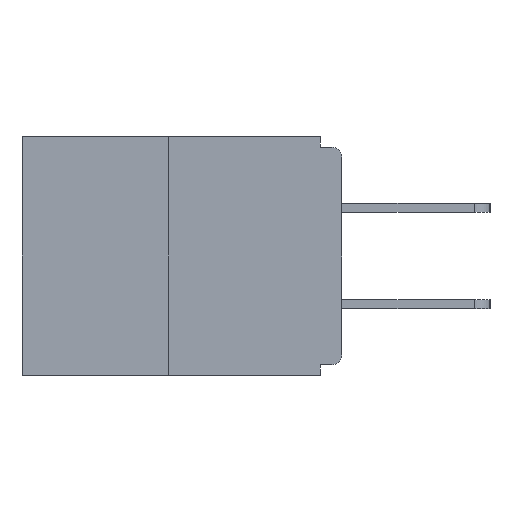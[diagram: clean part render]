
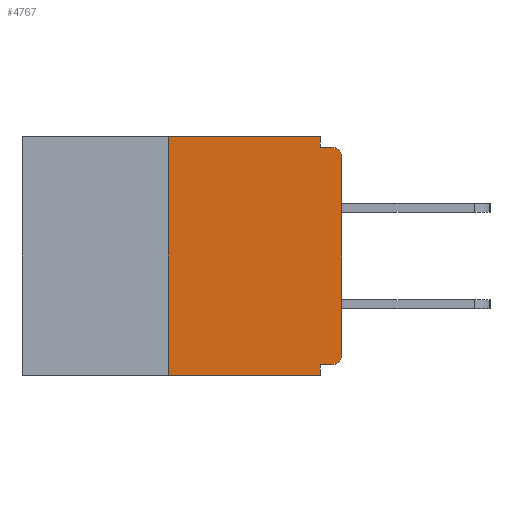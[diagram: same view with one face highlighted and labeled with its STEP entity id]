
A CAD part, left-side view. The second image highlights one B-rep face of the part: STEP entity #4767.
In plain terms, the highlighted planar face has unit normal (-1, 0, 0).
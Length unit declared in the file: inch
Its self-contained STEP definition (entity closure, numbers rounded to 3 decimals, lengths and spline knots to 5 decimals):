
#64 = EDGE_CURVE ( 'NONE', #5616, #4989, #21523, .T. ) ;
#118 = ORIENTED_EDGE ( 'NONE', *, *, #18176, .T. ) ;
#177 = VECTOR ( 'NONE', #8332, 39.37008 ) ;
#263 = EDGE_CURVE ( 'NONE', #3204, #12096, #264, .T. ) ;
#264 = LINE ( 'NONE', #6054, #12813 ) ;
#809 = CARTESIAN_POINT ( 'NONE',  ( 0., 0.015, -0.328 ) ) ;
#937 = DIRECTION ( 'NONE',  ( 0., 0., -1. ) ) ;
#1029 = CARTESIAN_POINT ( 'NONE',  ( 0., 0.015, -0.03 ) ) ;
#1104 = LINE ( 'NONE', #6964, #10248 ) ;
#1105 = EDGE_LOOP ( 'NONE', ( #10310, #10347, #118, #11314, #3718, #8852, #13658, #4213, #9443, #12826 ) ) ;
#1657 = VERTEX_POINT ( 'NONE', #8244 ) ;
#1823 = DIRECTION ( 'NONE',  ( 0., -1., 0. ) ) ;
#2028 = VERTEX_POINT ( 'NONE', #19215 ) ;
#2072 = CARTESIAN_POINT ( 'NONE',  ( 0., 0.46, -0.343 ) ) ;
#2690 = EDGE_CURVE ( 'NONE', #9528, #6956, #1104, .T. ) ;
#2830 = LINE ( 'NONE', #2072, #20263 ) ;
#3204 = VERTEX_POINT ( 'NONE', #15800 ) ;
#3490 = VECTOR ( 'NONE', #21428, 39.37008 ) ;
#3718 = ORIENTED_EDGE ( 'NONE', *, *, #64, .F. ) ;
#4213 = ORIENTED_EDGE ( 'NONE', *, *, #21224, .T. ) ;
#4306 = LINE ( 'NONE', #10295, #17257 ) ;
#4535 = LINE ( 'NONE', #6152, #3490 ) ;
#4767 = ADVANCED_FACE ( 'NONE', ( #7754 ), #18972, .F. ) ;
#4989 = VERTEX_POINT ( 'NONE', #6223 ) ;
#5616 = VERTEX_POINT ( 'NONE', #809 ) ;
#5651 = EDGE_CURVE ( 'NONE', #2028, #3204, #4535, .T. ) ;
#5868 = CARTESIAN_POINT ( 'NONE',  ( 0., 0.015, -0.313 ) ) ;
#6054 = CARTESIAN_POINT ( 'NONE',  ( 0., 0., -0.015 ) ) ;
#6152 = CARTESIAN_POINT ( 'NONE',  ( 0., 0.031, 0. ) ) ;
#6223 = CARTESIAN_POINT ( 'NONE',  ( 0., 0.031, -0.328 ) ) ;
#6956 = VERTEX_POINT ( 'NONE', #8049 ) ;
#6964 = CARTESIAN_POINT ( 'NONE',  ( 0., 0., 0. ) ) ;
#7022 = CARTESIAN_POINT ( 'NONE',  ( 0., 0.25, -0.343 ) ) ;
#7195 = EDGE_CURVE ( 'NONE', #4989, #18118, #16935, .T. ) ;
#7754 = FACE_OUTER_BOUND ( 'NONE', #1105, .T. ) ;
#8049 = CARTESIAN_POINT ( 'NONE',  ( 0., 0., -0.03 ) ) ;
#8244 = CARTESIAN_POINT ( 'NONE',  ( 0., 0.25, 0. ) ) ;
#8258 = CARTESIAN_POINT ( 'NONE',  ( 0., 0., -0.328 ) ) ;
#8332 = DIRECTION ( 'NONE',  ( 0., 0., 1. ) ) ;
#8852 = ORIENTED_EDGE ( 'NONE', *, *, #16119, .T. ) ;
#9039 = DIRECTION ( 'NONE',  ( 1., 0., 0. ) ) ;
#9443 = ORIENTED_EDGE ( 'NONE', *, *, #263, .F. ) ;
#9480 = CIRCLE ( 'NONE', #14640, 0.015 ) ;
#9528 = VERTEX_POINT ( 'NONE', #12200 ) ;
#9607 = CARTESIAN_POINT ( 'NONE',  ( 0., 0.031, -0.343 ) ) ;
#10248 = VECTOR ( 'NONE', #20206, 39.37008 ) ;
#10291 = AXIS2_PLACEMENT_3D ( 'NONE', #17436, #9039, #12404 ) ;
#10295 = CARTESIAN_POINT ( 'NONE',  ( 0., 0.46, 0. ) ) ;
#10310 = ORIENTED_EDGE ( 'NONE', *, *, #19624, .F. ) ;
#10347 = ORIENTED_EDGE ( 'NONE', *, *, #14015, .F. ) ;
#10361 = LINE ( 'NONE', #16898, #177 ) ;
#11125 = DIRECTION ( 'NONE',  ( 0., 0., -1. ) ) ;
#11220 = CIRCLE ( 'NONE', #15861, 0.015 ) ;
#11314 = ORIENTED_EDGE ( 'NONE', *, *, #7195, .F. ) ;
#11429 = DIRECTION ( 'NONE',  ( 0., 1., 0. ) ) ;
#12096 = VERTEX_POINT ( 'NONE', #20408 ) ;
#12200 = CARTESIAN_POINT ( 'NONE',  ( 0., 0., -0.313 ) ) ;
#12404 = DIRECTION ( 'NONE',  ( 0., 0., -1. ) ) ;
#12578 = DIRECTION ( 'NONE',  ( -1., 0., 0. ) ) ;
#12813 = VECTOR ( 'NONE', #19478, 39.37008 ) ;
#12826 = ORIENTED_EDGE ( 'NONE', *, *, #5651, .F. ) ;
#12933 = VERTEX_POINT ( 'NONE', #7022 ) ;
#13339 = CARTESIAN_POINT ( 'NONE',  ( 0., 0.031, -0.343 ) ) ;
#13628 = VECTOR ( 'NONE', #11429, 39.37008 ) ;
#13658 = ORIENTED_EDGE ( 'NONE', *, *, #2690, .T. ) ;
#14015 = EDGE_CURVE ( 'NONE', #12933, #1657, #10361, .T. ) ;
#14640 = AXIS2_PLACEMENT_3D ( 'NONE', #5868, #12578, #937 ) ;
#15770 = DIRECTION ( 'NONE',  ( 0., -1., 0. ) ) ;
#15800 = CARTESIAN_POINT ( 'NONE',  ( 0., 0.031, -0.015 ) ) ;
#15861 = AXIS2_PLACEMENT_3D ( 'NONE', #1029, #21172, #11125 ) ;
#16119 = EDGE_CURVE ( 'NONE', #5616, #9528, #9480, .T. ) ;
#16343 = DIRECTION ( 'NONE',  ( 0., 0., -1. ) ) ;
#16898 = CARTESIAN_POINT ( 'NONE',  ( 0., 0.25, 0. ) ) ;
#16935 = LINE ( 'NONE', #9607, #19281 ) ;
#17257 = VECTOR ( 'NONE', #1823, 39.37008 ) ;
#17436 = CARTESIAN_POINT ( 'NONE',  ( 0., 0.46, 0. ) ) ;
#18118 = VERTEX_POINT ( 'NONE', #13339 ) ;
#18176 = EDGE_CURVE ( 'NONE', #12933, #18118, #2830, .T. ) ;
#18972 = PLANE ( 'NONE',  #10291 ) ;
#19215 = CARTESIAN_POINT ( 'NONE',  ( 0., 0.031, 0. ) ) ;
#19281 = VECTOR ( 'NONE', #16343, 39.37008 ) ;
#19478 = DIRECTION ( 'NONE',  ( 0., -1., 0. ) ) ;
#19624 = EDGE_CURVE ( 'NONE', #1657, #2028, #4306, .T. ) ;
#20206 = DIRECTION ( 'NONE',  ( 0., 0., 1. ) ) ;
#20263 = VECTOR ( 'NONE', #15770, 39.37008 ) ;
#20408 = CARTESIAN_POINT ( 'NONE',  ( 0., 0.015, -0.015 ) ) ;
#21172 = DIRECTION ( 'NONE',  ( -1., 0., 0. ) ) ;
#21224 = EDGE_CURVE ( 'NONE', #6956, #12096, #11220, .T. ) ;
#21428 = DIRECTION ( 'NONE',  ( 0., 0., -1. ) ) ;
#21523 = LINE ( 'NONE', #8258, #13628 ) ;
